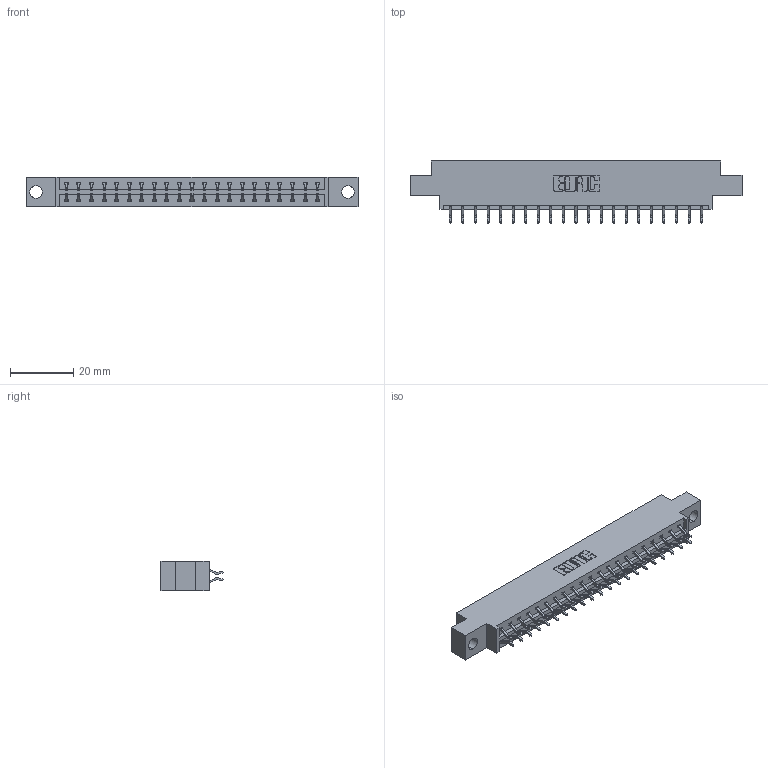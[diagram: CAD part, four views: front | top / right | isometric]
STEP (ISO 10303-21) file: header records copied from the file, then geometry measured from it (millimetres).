
FILE_DESCRIPTION (( 'STEP AP203' ), '1' );
FILE_NAME ('833-042-556-804.STEP', '2020-06-03T22:22:50', ( '' ), ( '' ), 'SwSTEP 2.0', 'SolidWorks 2020', '' );
FILE_SCHEMA (( 'CONFIG_CONTROL_DESIGN' ));
Length unit declared in the file: inch
Products named in the file (3): 345-292-001_556 Tail; 833-042-556-804; 833 Part_Offset - .156 Dia - TH
Assembly tree (43 placements, depth 2):
  833-042-556-804
    833 Part_Offset - .156 Dia - TH
    345-292-001_556 Tail  x42
Bounding box: 104.75 x 19.57 x 9.4 mm (x, y, z)
Volume: 10180.6 mm3; surface area: 11789.2 mm2
Topology: 43 solids, 43 shells, 2554 faces, 7589 edges, 5002 vertices
Faces by surface type: plane 1754, cylinder 800
Entity records: 16581 total; most frequent: CARTESIAN_POINT 2790, ORIENTED_EDGE 2714, DIRECTION 2409, EDGE_CURVE 1357, VECTOR 1221, LINE 1221, VERTEX_POINT 902, AXIS2_PLACEMENT_3D 594
